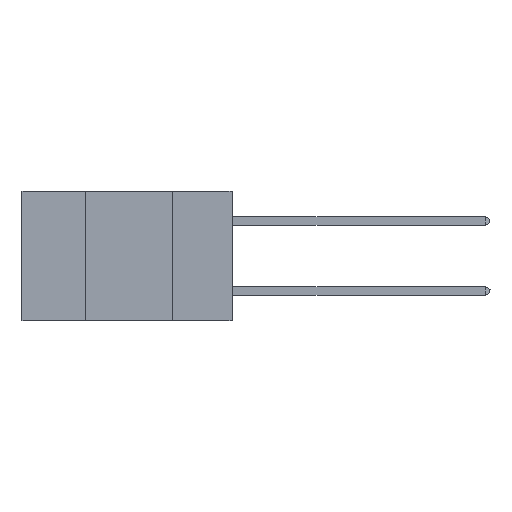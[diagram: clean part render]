
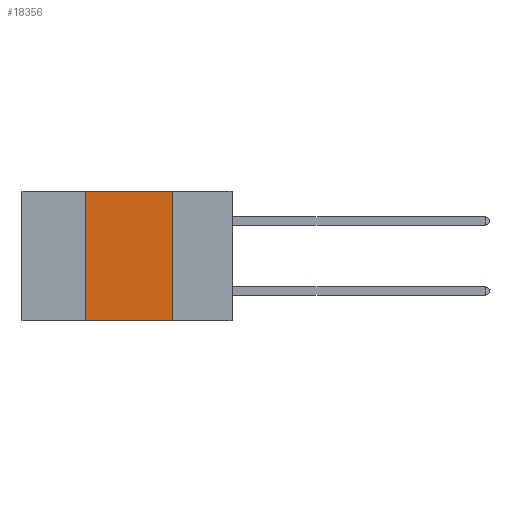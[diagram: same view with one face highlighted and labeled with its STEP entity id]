
A CAD part, left-side view. The second image highlights one B-rep face of the part: STEP entity #18356.
In plain terms, the highlighted planar face has unit normal (-1, 0, 0).
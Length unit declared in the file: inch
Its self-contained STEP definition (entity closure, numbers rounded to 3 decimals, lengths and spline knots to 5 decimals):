
#105 = VECTOR ( 'NONE', #21248, 39.37008 ) ;
#472 = CARTESIAN_POINT ( 'NONE',  ( 0., 0.17, 0. ) ) ;
#1338 = ORIENTED_EDGE ( 'NONE', *, *, #11047, .F. ) ;
#1749 = DIRECTION ( 'NONE',  ( 0., 0., -1. ) ) ;
#2903 = VERTEX_POINT ( 'NONE', #15814 ) ;
#4293 = ORIENTED_EDGE ( 'NONE', *, *, #7241, .F. ) ;
#4623 = DIRECTION ( 'NONE',  ( 0., -1., 0. ) ) ;
#4752 = LINE ( 'NONE', #21084, #105 ) ;
#4778 = LINE ( 'NONE', #12624, #23936 ) ;
#4826 = VERTEX_POINT ( 'NONE', #472 ) ;
#5474 = FACE_OUTER_BOUND ( 'NONE', #12096, .T. ) ;
#5529 = CARTESIAN_POINT ( 'NONE',  ( 0., 0.6, 0. ) ) ;
#7138 = CARTESIAN_POINT ( 'NONE',  ( 0., 0.42, 0. ) ) ;
#7241 = EDGE_CURVE ( 'NONE', #4826, #14997, #14803, .T. ) ;
#7817 = VERTEX_POINT ( 'NONE', #7138 ) ;
#8201 = CARTESIAN_POINT ( 'NONE',  ( 0., 0.17, 0. ) ) ;
#9232 = PLANE ( 'NONE',  #14483 ) ;
#9570 = ORIENTED_EDGE ( 'NONE', *, *, #21288, .T. ) ;
#10181 = DIRECTION ( 'NONE',  ( 0., 0., -1. ) ) ;
#11047 = EDGE_CURVE ( 'NONE', #2903, #7817, #12216, .T. ) ;
#11291 = ORIENTED_EDGE ( 'NONE', *, *, #21768, .F. ) ;
#11354 = CARTESIAN_POINT ( 'NONE',  ( 0., 0.42, 0. ) ) ;
#12096 = EDGE_LOOP ( 'NONE', ( #4293, #11291, #1338, #9570 ) ) ;
#12216 = LINE ( 'NONE', #11354, #17169 ) ;
#12624 = CARTESIAN_POINT ( 'NONE',  ( 0., 0.6, -0.37 ) ) ;
#14483 = AXIS2_PLACEMENT_3D ( 'NONE', #5529, #22022, #1749 ) ;
#14803 = LINE ( 'NONE', #8201, #20352 ) ;
#14997 = VERTEX_POINT ( 'NONE', #22369 ) ;
#15814 = CARTESIAN_POINT ( 'NONE',  ( 0., 0.42, -0.37 ) ) ;
#17169 = VECTOR ( 'NONE', #18827, 39.37008 ) ;
#18356 = ADVANCED_FACE ( 'NONE', ( #5474 ), #9232, .F. ) ;
#18827 = DIRECTION ( 'NONE',  ( 0., 0., 1. ) ) ;
#20352 = VECTOR ( 'NONE', #10181, 39.37008 ) ;
#21084 = CARTESIAN_POINT ( 'NONE',  ( 0., 0.6, 0. ) ) ;
#21248 = DIRECTION ( 'NONE',  ( 0., -1., 0. ) ) ;
#21288 = EDGE_CURVE ( 'NONE', #2903, #14997, #4778, .T. ) ;
#21768 = EDGE_CURVE ( 'NONE', #7817, #4826, #4752, .T. ) ;
#22022 = DIRECTION ( 'NONE',  ( 1., 0., 0. ) ) ;
#22369 = CARTESIAN_POINT ( 'NONE',  ( 0., 0.17, -0.37 ) ) ;
#23936 = VECTOR ( 'NONE', #4623, 39.37008 ) ;
